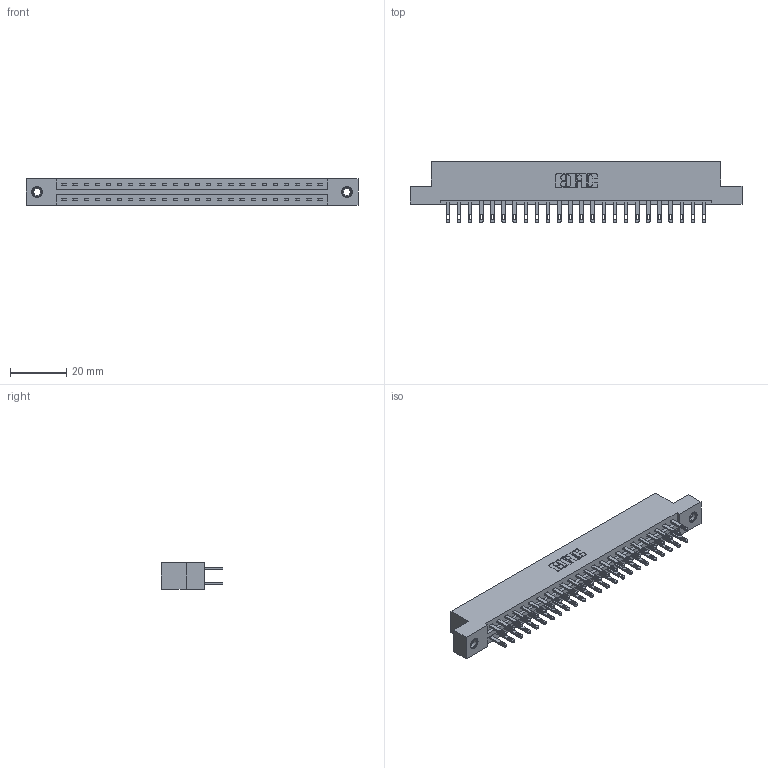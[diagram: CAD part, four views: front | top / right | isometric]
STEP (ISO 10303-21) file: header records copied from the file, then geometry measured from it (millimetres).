
FILE_DESCRIPTION (( 'STEP AP203' ), '1' );
FILE_NAME ('887-048-500-207.STEP', '2020-09-21T00:53:12', ( '' ), ( '' ), 'SwSTEP 2.0', 'SolidWorks 2020', '' );
FILE_SCHEMA (( 'CONFIG_CONTROL_DESIGN' ));
Length unit declared in the file: inch
Products named in the file (4): 345-292-001_345-293-100; 887-048-500-207; 837 Part_Flush Mounting Lugs - 0.156 Dia-TI; 345-250-001_345-250-005-103
Assembly tree (51 placements, depth 2):
  887-048-500-207
    837 Part_Flush Mounting Lugs - 0.156 Dia-TI
    345-292-001_345-293-100  x48
    345-250-001_345-250-005-103  x2
Bounding box: 118.11 x 21.85 x 9.4 mm (x, y, z)
Volume: 12340.9 mm3; surface area: 14345.1 mm2
Topology: 51 solids, 51 shells, 2574 faces, 7791 edges, 5186 vertices
Faces by surface type: plane 1638, cylinder 920, cone 12, torus 4
Entity records: 22052 total; most frequent: CARTESIAN_POINT 3709, ORIENTED_EDGE 3638, DIRECTION 3221, EDGE_CURVE 1819, VECTOR 1667, LINE 1667, VERTEX_POINT 1208, AXIS2_PLACEMENT_3D 777
